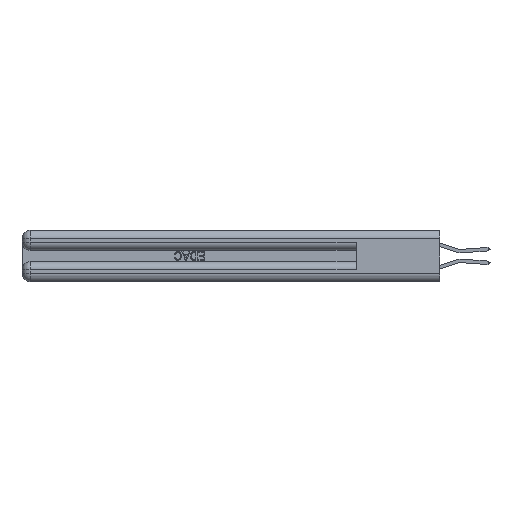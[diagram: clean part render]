
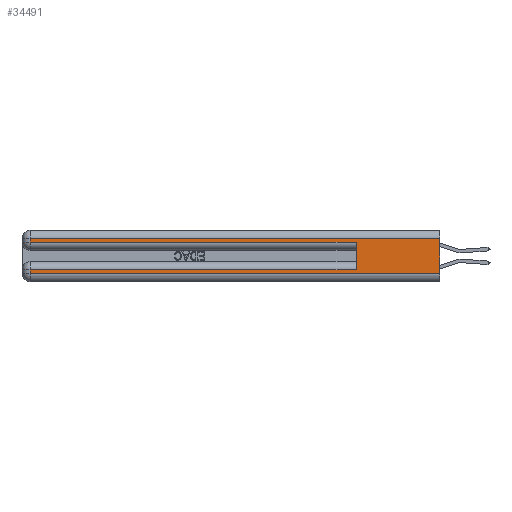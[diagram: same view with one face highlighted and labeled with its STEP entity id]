
A CAD part, left-side view. The second image highlights one B-rep face of the part: STEP entity #34491.
In plain terms, the highlighted planar face has unit normal (-1, 0, 0).
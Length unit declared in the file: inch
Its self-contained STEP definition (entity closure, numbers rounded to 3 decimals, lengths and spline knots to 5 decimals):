
#1274 = CARTESIAN_POINT ( 'NONE',  ( 0., 2.94, 0.37 ) ) ;
#2511 = DIRECTION ( 'NONE',  ( 0., 0., 1. ) ) ;
#4095 = CARTESIAN_POINT ( 'NONE',  ( 0., 2.94, 0.085 ) ) ;
#4147 = CARTESIAN_POINT ( 'NONE',  ( 0., 0.6, 0.285 ) ) ;
#5778 = ORIENTED_EDGE ( 'NONE', *, *, #34956, .T. ) ;
#6032 = EDGE_CURVE ( 'NONE', #23151, #20389, #22812, .T. ) ;
#6355 = CARTESIAN_POINT ( 'NONE',  ( 0., 0., 0.31 ) ) ;
#7653 = EDGE_CURVE ( 'NONE', #8734, #20389, #15016, .T. ) ;
#7775 = VECTOR ( 'NONE', #38723, 39.37008 ) ;
#7780 = LINE ( 'NONE', #10257, #23102 ) ;
#8385 = CARTESIAN_POINT ( 'NONE',  ( 0., 0., 0.06 ) ) ;
#8390 = VECTOR ( 'NONE', #18242, 39.37008 ) ;
#8734 = VERTEX_POINT ( 'NONE', #35523 ) ;
#9109 = ORIENTED_EDGE ( 'NONE', *, *, #12518, .F. ) ;
#9242 = EDGE_CURVE ( 'NONE', #12901, #8734, #7780, .T. ) ;
#9529 = LINE ( 'NONE', #6355, #24837 ) ;
#10257 = CARTESIAN_POINT ( 'NONE',  ( 0., 2.94, 0.37 ) ) ;
#10406 = CARTESIAN_POINT ( 'NONE',  ( 0., 0., 0.285 ) ) ;
#11112 = VERTEX_POINT ( 'NONE', #37614 ) ;
#11728 = CARTESIAN_POINT ( 'NONE',  ( 0., 0., 0.31 ) ) ;
#12503 = DIRECTION ( 'NONE',  ( 0., 1., 0. ) ) ;
#12518 = EDGE_CURVE ( 'NONE', #28777, #16538, #24054, .T. ) ;
#12809 = LINE ( 'NONE', #8385, #35268 ) ;
#12901 = VERTEX_POINT ( 'NONE', #28348 ) ;
#13335 = DIRECTION ( 'NONE',  ( 0., 0., -1. ) ) ;
#14401 = DIRECTION ( 'NONE',  ( 1., 0., 0. ) ) ;
#14674 = VECTOR ( 'NONE', #2511, 39.37008 ) ;
#15016 = LINE ( 'NONE', #10406, #29382 ) ;
#15805 = ORIENTED_EDGE ( 'NONE', *, *, #34530, .T. ) ;
#16538 = VERTEX_POINT ( 'NONE', #29144 ) ;
#17210 = ORIENTED_EDGE ( 'NONE', *, *, #23014, .T. ) ;
#17597 = DIRECTION ( 'NONE',  ( 0., -1., 0. ) ) ;
#17918 = EDGE_LOOP ( 'NONE', ( #9109, #17210, #19173, #35400, #20135, #21084, #5778, #15805 ) ) ;
#18242 = DIRECTION ( 'NONE',  ( 0., 1., 0. ) ) ;
#18429 = EDGE_CURVE ( 'NONE', #23151, #32979, #23719, .T. ) ;
#19173 = ORIENTED_EDGE ( 'NONE', *, *, #9242, .T. ) ;
#19611 = DIRECTION ( 'NONE',  ( 0., 0., -1. ) ) ;
#20135 = ORIENTED_EDGE ( 'NONE', *, *, #6032, .F. ) ;
#20389 = VERTEX_POINT ( 'NONE', #4147 ) ;
#21084 = ORIENTED_EDGE ( 'NONE', *, *, #18429, .T. ) ;
#22812 = LINE ( 'NONE', #26307, #14674 ) ;
#23014 = EDGE_CURVE ( 'NONE', #28777, #12901, #9529, .T. ) ;
#23102 = VECTOR ( 'NONE', #13335, 39.37008 ) ;
#23151 = VERTEX_POINT ( 'NONE', #25343 ) ;
#23508 = CARTESIAN_POINT ( 'NONE',  ( 0., 0., 0.37 ) ) ;
#23547 = CARTESIAN_POINT ( 'NONE',  ( 0., 0., 0.37 ) ) ;
#23719 = LINE ( 'NONE', #33467, #8390 ) ;
#24054 = LINE ( 'NONE', #23547, #7775 ) ;
#24837 = VECTOR ( 'NONE', #12503, 39.37008 ) ;
#25343 = CARTESIAN_POINT ( 'NONE',  ( 0., 0.6, 0.085 ) ) ;
#26307 = CARTESIAN_POINT ( 'NONE',  ( 0., 0.6, 0.145 ) ) ;
#28101 = LINE ( 'NONE', #1274, #35232 ) ;
#28348 = CARTESIAN_POINT ( 'NONE',  ( 0., 2.94, 0.31 ) ) ;
#28777 = VERTEX_POINT ( 'NONE', #11728 ) ;
#29091 = FACE_OUTER_BOUND ( 'NONE', #17918, .T. ) ;
#29144 = CARTESIAN_POINT ( 'NONE',  ( 0., 0., 0.06 ) ) ;
#29382 = VECTOR ( 'NONE', #34860, 39.37008 ) ;
#32713 = PLANE ( 'NONE',  #39140 ) ;
#32979 = VERTEX_POINT ( 'NONE', #4095 ) ;
#33467 = CARTESIAN_POINT ( 'NONE',  ( 0., 0., 0.085 ) ) ;
#34491 = ADVANCED_FACE ( 'NONE', ( #29091 ), #32713, .F. ) ;
#34530 = EDGE_CURVE ( 'NONE', #11112, #16538, #12809, .T. ) ;
#34860 = DIRECTION ( 'NONE',  ( 0., -1., 0. ) ) ;
#34956 = EDGE_CURVE ( 'NONE', #32979, #11112, #28101, .T. ) ;
#35232 = VECTOR ( 'NONE', #19611, 39.37008 ) ;
#35268 = VECTOR ( 'NONE', #17597, 39.37008 ) ;
#35400 = ORIENTED_EDGE ( 'NONE', *, *, #7653, .T. ) ;
#35523 = CARTESIAN_POINT ( 'NONE',  ( 0., 2.94, 0.285 ) ) ;
#35764 = DIRECTION ( 'NONE',  ( 0., 0., -1. ) ) ;
#37614 = CARTESIAN_POINT ( 'NONE',  ( 0., 2.94, 0.06 ) ) ;
#38723 = DIRECTION ( 'NONE',  ( 0., 0., -1. ) ) ;
#39140 = AXIS2_PLACEMENT_3D ( 'NONE', #23508, #14401, #35764 ) ;
